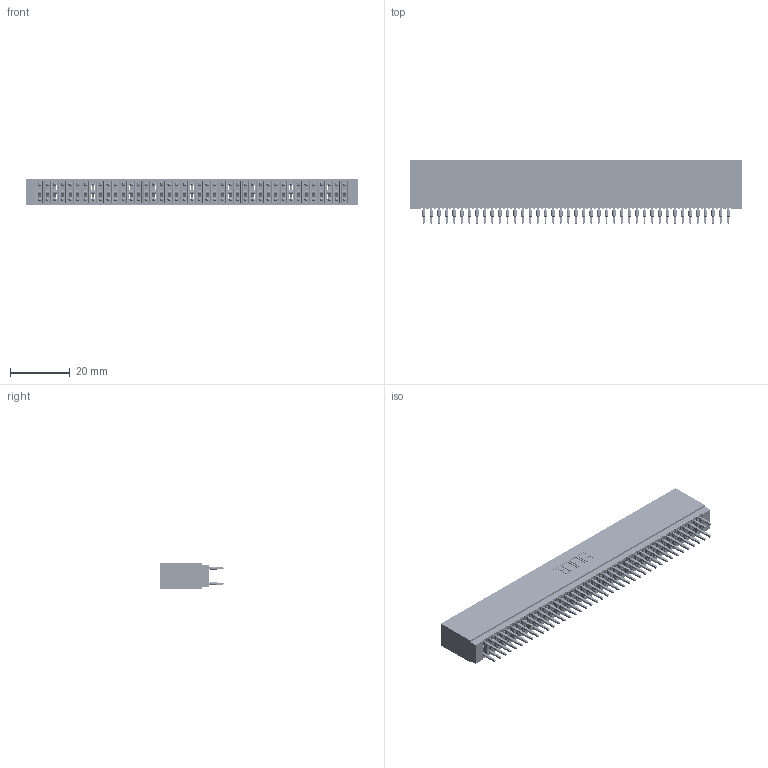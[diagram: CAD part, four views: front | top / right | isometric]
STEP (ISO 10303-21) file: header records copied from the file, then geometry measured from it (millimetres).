
FILE_DESCRIPTION (( 'STEP AP203' ), '1' );
FILE_NAME ('745-082-560-201.STEP', '2026-02-26T21:50:25', ( '' ), ( '' ), 'SwSTEP 2.0', 'SolidWorks 2023', '' );
FILE_SCHEMA (( 'CONFIG_CONTROL_DESIGN' ));
Length unit declared in the file: millimetre
Products named in the file (3): 745-082-560-201; 745 Part_Insulator Option - 01; 745-292-001_560
Assembly tree (83 placements, depth 2):
  745-082-560-201
    745 Part_Insulator Option - 01
    745-292-001_560  x82
Bounding box: 110.74 x 21.22 x 8.89 mm (x, y, z)
Volume: 10283.1 mm3; surface area: 22174.5 mm2
Topology: 83 solids, 83 shells, 8172 faces, 22357 edges, 14194 vertices
Faces by surface type: plane 4237, cylinder 1803, bspline 1640, torus 492
Entity records: 69484 total; most frequent: CARTESIAN_POINT 12557, ORIENTED_EDGE 11990, DIRECTION 10479, EDGE_CURVE 5995, LINE 5559, VECTOR 5559, VERTEX_POINT 3826, AXIS2_PLACEMENT_3D 2460
